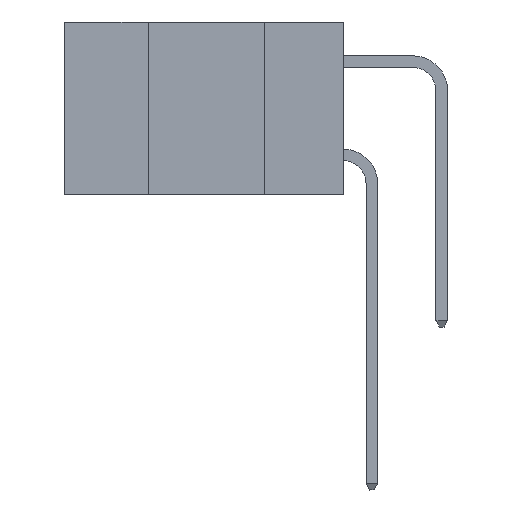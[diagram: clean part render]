
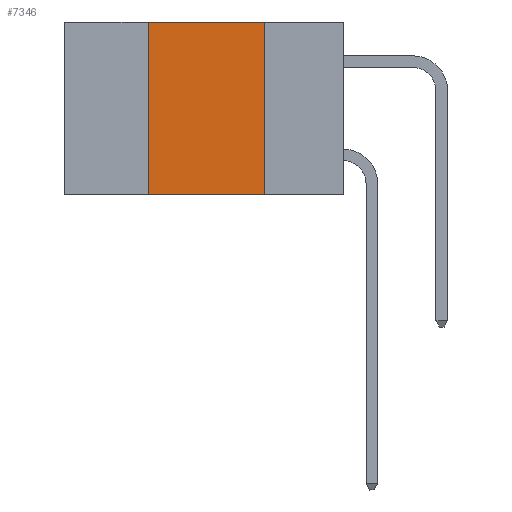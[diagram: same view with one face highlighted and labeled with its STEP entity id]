
A CAD part, left-side view. The second image highlights one B-rep face of the part: STEP entity #7346.
In plain terms, the highlighted planar face has unit normal (-1, 0, 0).
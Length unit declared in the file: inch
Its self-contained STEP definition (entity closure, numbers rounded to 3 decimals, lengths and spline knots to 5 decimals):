
#288 = VERTEX_POINT ( 'NONE', #3848 ) ;
#1047 = VECTOR ( 'NONE', #11780, 39.37008 ) ;
#1423 = FACE_OUTER_BOUND ( 'NONE', #16500, .T. ) ;
#2071 = AXIS2_PLACEMENT_3D ( 'NONE', #4550, #4495, #4434 ) ;
#2211 = ORIENTED_EDGE ( 'NONE', *, *, #8703, .T. ) ;
#2337 = VERTEX_POINT ( 'NONE', #10525 ) ;
#2932 = VERTEX_POINT ( 'NONE', #10040 ) ;
#3206 = VECTOR ( 'NONE', #8493, 39.37008 ) ;
#3848 = CARTESIAN_POINT ( 'NONE',  ( 0., 0.42, 0. ) ) ;
#4407 = CARTESIAN_POINT ( 'NONE',  ( 0., 0.17, 0. ) ) ;
#4434 = DIRECTION ( 'NONE',  ( 0., 0., -1. ) ) ;
#4495 = DIRECTION ( 'NONE',  ( 1., 0., 0. ) ) ;
#4550 = CARTESIAN_POINT ( 'NONE',  ( 0., 0.6, 0. ) ) ;
#4632 = PLANE ( 'NONE',  #2071 ) ;
#4941 = ORIENTED_EDGE ( 'NONE', *, *, #8902, .F. ) ;
#7346 = ADVANCED_FACE ( 'NONE', ( #1423 ), #4632, .F. ) ;
#8493 = DIRECTION ( 'NONE',  ( 0., 0., -1. ) ) ;
#8703 = EDGE_CURVE ( 'NONE', #2337, #2932, #16760, .T. ) ;
#8757 = CARTESIAN_POINT ( 'NONE',  ( 0., 0.17, -0.37 ) ) ;
#8859 = VECTOR ( 'NONE', #10914, 39.37008 ) ;
#8902 = EDGE_CURVE ( 'NONE', #15509, #2932, #15141, .T. ) ;
#9243 = EDGE_CURVE ( 'NONE', #2337, #288, #13274, .T. ) ;
#9354 = DIRECTION ( 'NONE',  ( 0., -1., 0. ) ) ;
#9609 = ORIENTED_EDGE ( 'NONE', *, *, #9243, .F. ) ;
#10040 = CARTESIAN_POINT ( 'NONE',  ( 0., 0.17, -0.37 ) ) ;
#10525 = CARTESIAN_POINT ( 'NONE',  ( 0., 0.42, -0.37 ) ) ;
#10615 = VECTOR ( 'NONE', #9354, 39.37008 ) ;
#10914 = DIRECTION ( 'NONE',  ( 0., 0., 1. ) ) ;
#11780 = DIRECTION ( 'NONE',  ( 0., -1., 0. ) ) ;
#11788 = CARTESIAN_POINT ( 'NONE',  ( 0., 0.6, 0. ) ) ;
#12155 = EDGE_CURVE ( 'NONE', #288, #15509, #15434, .T. ) ;
#12789 = CARTESIAN_POINT ( 'NONE',  ( 0., 0.42, -0.37 ) ) ;
#13274 = LINE ( 'NONE', #12789, #8859 ) ;
#13618 = CARTESIAN_POINT ( 'NONE',  ( 0., 0.6, -0.37 ) ) ;
#15141 = LINE ( 'NONE', #8757, #3206 ) ;
#15434 = LINE ( 'NONE', #11788, #1047 ) ;
#15509 = VERTEX_POINT ( 'NONE', #4407 ) ;
#16406 = ORIENTED_EDGE ( 'NONE', *, *, #12155, .F. ) ;
#16500 = EDGE_LOOP ( 'NONE', ( #4941, #16406, #9609, #2211 ) ) ;
#16760 = LINE ( 'NONE', #13618, #10615 ) ;
